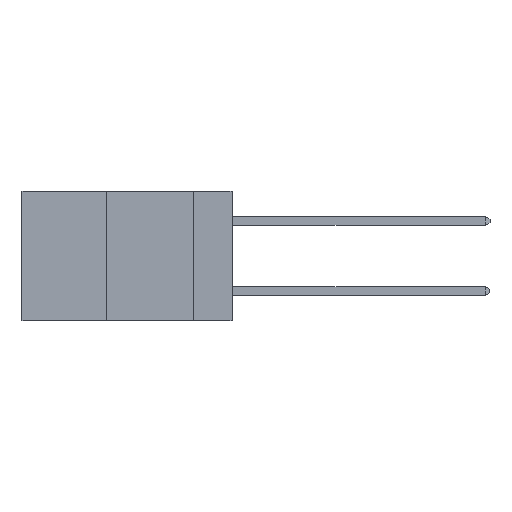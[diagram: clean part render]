
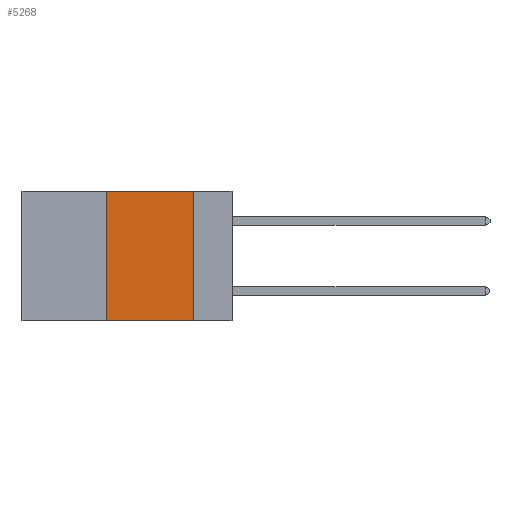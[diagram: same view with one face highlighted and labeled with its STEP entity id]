
A CAD part, left-side view. The second image highlights one B-rep face of the part: STEP entity #5268.
In plain terms, the highlighted planar face has unit normal (-1, 0, 0).
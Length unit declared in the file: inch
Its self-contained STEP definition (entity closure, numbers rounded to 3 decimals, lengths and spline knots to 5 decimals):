
#1012 = VERTEX_POINT ( 'NONE', #15954 ) ;
#1328 = CARTESIAN_POINT ( 'NONE',  ( 0., 0.6, 0. ) ) ;
#1417 = VECTOR ( 'NONE', #4111, 39.37008 ) ;
#2459 = CARTESIAN_POINT ( 'NONE',  ( 0., 0.36, 0. ) ) ;
#2765 = LINE ( 'NONE', #16275, #3267 ) ;
#2922 = CARTESIAN_POINT ( 'NONE',  ( 0., 0.6, -0.37 ) ) ;
#3163 = ORIENTED_EDGE ( 'NONE', *, *, #17908, .F. ) ;
#3267 = VECTOR ( 'NONE', #13260, 39.37008 ) ;
#4111 = DIRECTION ( 'NONE',  ( 0., 0., 1. ) ) ;
#4374 = DIRECTION ( 'NONE',  ( 1., 0., 0. ) ) ;
#4580 = DIRECTION ( 'NONE',  ( 0., -1., 0. ) ) ;
#4586 = CARTESIAN_POINT ( 'NONE',  ( 0., 0.36, -0.37 ) ) ;
#5106 = LINE ( 'NONE', #2922, #8237 ) ;
#5268 = ADVANCED_FACE ( 'NONE', ( #11141 ), #13567, .F. ) ;
#5338 = EDGE_CURVE ( 'NONE', #8626, #9171, #5106, .T. ) ;
#6577 = EDGE_CURVE ( 'NONE', #16896, #1012, #9263, .T. ) ;
#7391 = CARTESIAN_POINT ( 'NONE',  ( 0., 0.6, 0. ) ) ;
#8237 = VECTOR ( 'NONE', #4580, 39.37008 ) ;
#8626 = VERTEX_POINT ( 'NONE', #4586 ) ;
#9171 = VERTEX_POINT ( 'NONE', #13412 ) ;
#9263 = LINE ( 'NONE', #1328, #12847 ) ;
#10402 = AXIS2_PLACEMENT_3D ( 'NONE', #7391, #4374, #15077 ) ;
#10576 = ORIENTED_EDGE ( 'NONE', *, *, #5338, .T. ) ;
#10751 = ORIENTED_EDGE ( 'NONE', *, *, #19844, .F. ) ;
#11058 = ORIENTED_EDGE ( 'NONE', *, *, #6577, .F. ) ;
#11141 = FACE_OUTER_BOUND ( 'NONE', #14759, .T. ) ;
#12847 = VECTOR ( 'NONE', #16786, 39.37008 ) ;
#13260 = DIRECTION ( 'NONE',  ( 0., 0., -1. ) ) ;
#13412 = CARTESIAN_POINT ( 'NONE',  ( 0., 0.11, -0.37 ) ) ;
#13567 = PLANE ( 'NONE',  #10402 ) ;
#14759 = EDGE_LOOP ( 'NONE', ( #3163, #11058, #10751, #10576 ) ) ;
#15077 = DIRECTION ( 'NONE',  ( 0., 0., -1. ) ) ;
#15954 = CARTESIAN_POINT ( 'NONE',  ( 0., 0.11, 0. ) ) ;
#16275 = CARTESIAN_POINT ( 'NONE',  ( 0., 0.11, 0. ) ) ;
#16786 = DIRECTION ( 'NONE',  ( 0., -1., 0. ) ) ;
#16896 = VERTEX_POINT ( 'NONE', #18787 ) ;
#17338 = LINE ( 'NONE', #2459, #1417 ) ;
#17908 = EDGE_CURVE ( 'NONE', #1012, #9171, #2765, .T. ) ;
#18787 = CARTESIAN_POINT ( 'NONE',  ( 0., 0.36, 0. ) ) ;
#19844 = EDGE_CURVE ( 'NONE', #8626, #16896, #17338, .T. ) ;
